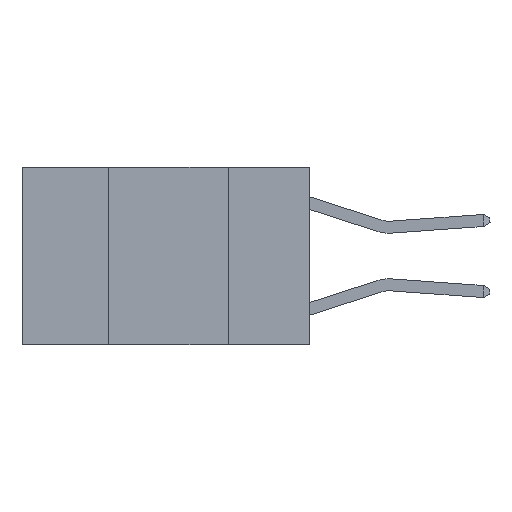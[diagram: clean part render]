
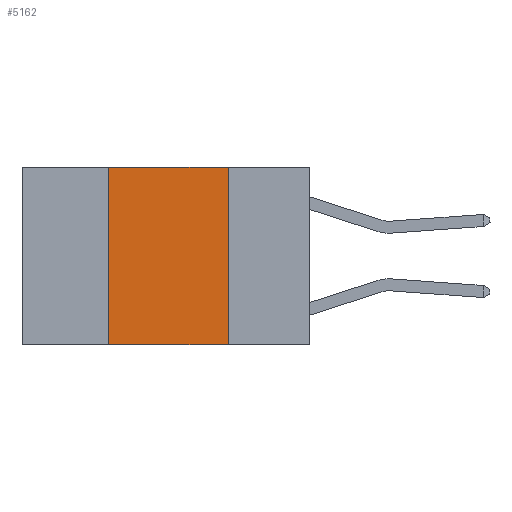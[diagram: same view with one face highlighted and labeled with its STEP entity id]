
A CAD part, left-side view. The second image highlights one B-rep face of the part: STEP entity #5162.
In plain terms, the highlighted planar face has unit normal (-1, 0, 0).
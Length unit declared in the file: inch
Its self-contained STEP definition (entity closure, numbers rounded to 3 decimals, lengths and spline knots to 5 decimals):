
#108 = DIRECTION ( 'NONE',  ( 0., 0., 1. ) ) ;
#250 = ORIENTED_EDGE ( 'NONE', *, *, #1722, .F. ) ;
#297 = CARTESIAN_POINT ( 'NONE',  ( 0., 0.17, 0. ) ) ;
#694 = CARTESIAN_POINT ( 'NONE',  ( 0., 0.17, 0. ) ) ;
#942 = EDGE_LOOP ( 'NONE', ( #250, #5050, #8780, #5738 ) ) ;
#1074 = LINE ( 'NONE', #7600, #9107 ) ;
#1722 = EDGE_CURVE ( 'NONE', #3804, #3111, #8910, .T. ) ;
#2001 = VECTOR ( 'NONE', #9390, 39.37008 ) ;
#2109 = LINE ( 'NONE', #6599, #7883 ) ;
#2751 = VECTOR ( 'NONE', #7960, 39.37008 ) ;
#2876 = EDGE_CURVE ( 'NONE', #3726, #3804, #1074, .T. ) ;
#3111 = VERTEX_POINT ( 'NONE', #3802 ) ;
#3163 = DIRECTION ( 'NONE',  ( 1., 0., 0. ) ) ;
#3533 = CARTESIAN_POINT ( 'NONE',  ( 0., 0.42, 0. ) ) ;
#3726 = VERTEX_POINT ( 'NONE', #3533 ) ;
#3802 = CARTESIAN_POINT ( 'NONE',  ( 0., 0.17, -0.37 ) ) ;
#3804 = VERTEX_POINT ( 'NONE', #297 ) ;
#4210 = VERTEX_POINT ( 'NONE', #6385 ) ;
#5050 = ORIENTED_EDGE ( 'NONE', *, *, #2876, .F. ) ;
#5162 = ADVANCED_FACE ( 'NONE', ( #8770 ), #6325, .F. ) ;
#5738 = ORIENTED_EDGE ( 'NONE', *, *, #7326, .T. ) ;
#5755 = CARTESIAN_POINT ( 'NONE',  ( 0., 0.6, -0.37 ) ) ;
#6325 = PLANE ( 'NONE',  #8714 ) ;
#6385 = CARTESIAN_POINT ( 'NONE',  ( 0., 0.42, -0.37 ) ) ;
#6509 = LINE ( 'NONE', #5755, #2001 ) ;
#6599 = CARTESIAN_POINT ( 'NONE',  ( 0., 0.42, 0. ) ) ;
#7326 = EDGE_CURVE ( 'NONE', #4210, #3111, #6509, .T. ) ;
#7600 = CARTESIAN_POINT ( 'NONE',  ( 0., 0.6, 0. ) ) ;
#7850 = CARTESIAN_POINT ( 'NONE',  ( 0., 0.6, 0. ) ) ;
#7883 = VECTOR ( 'NONE', #108, 39.37008 ) ;
#7960 = DIRECTION ( 'NONE',  ( 0., 0., -1. ) ) ;
#8223 = EDGE_CURVE ( 'NONE', #4210, #3726, #2109, .T. ) ;
#8610 = DIRECTION ( 'NONE',  ( 0., 0., -1. ) ) ;
#8714 = AXIS2_PLACEMENT_3D ( 'NONE', #7850, #3163, #8610 ) ;
#8770 = FACE_OUTER_BOUND ( 'NONE', #942, .T. ) ;
#8780 = ORIENTED_EDGE ( 'NONE', *, *, #8223, .F. ) ;
#8910 = LINE ( 'NONE', #694, #2751 ) ;
#9045 = DIRECTION ( 'NONE',  ( 0., -1., 0. ) ) ;
#9107 = VECTOR ( 'NONE', #9045, 39.37008 ) ;
#9390 = DIRECTION ( 'NONE',  ( 0., -1., 0. ) ) ;
